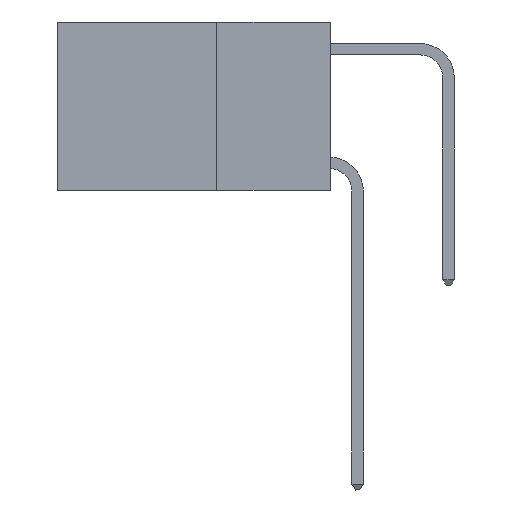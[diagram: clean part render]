
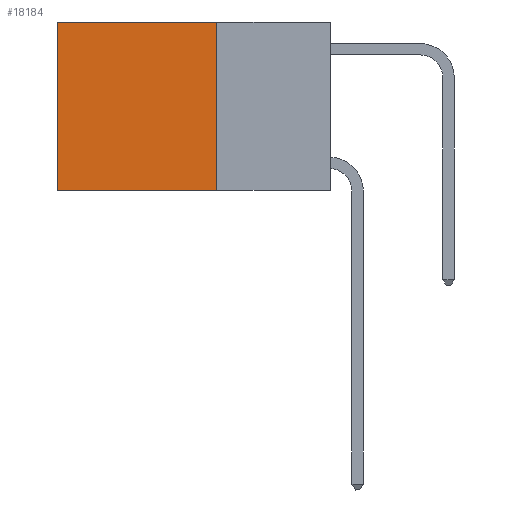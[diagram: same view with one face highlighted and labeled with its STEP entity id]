
A CAD part, left-side view. The second image highlights one B-rep face of the part: STEP entity #18184.
In plain terms, the highlighted planar face has unit normal (-1, 0, 0).
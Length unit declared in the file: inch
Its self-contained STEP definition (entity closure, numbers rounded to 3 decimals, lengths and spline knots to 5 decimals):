
#187 = ORIENTED_EDGE ( 'NONE', *, *, #11373, .F. ) ;
#1562 = VECTOR ( 'NONE', #7530, 39.37008 ) ;
#2436 = VERTEX_POINT ( 'NONE', #14082 ) ;
#2624 = AXIS2_PLACEMENT_3D ( 'NONE', #4639, #6409, #18191 ) ;
#2731 = EDGE_CURVE ( 'NONE', #2436, #19202, #10672, .T. ) ;
#3174 = EDGE_CURVE ( 'NONE', #18540, #13599, #18508, .T. ) ;
#4070 = CARTESIAN_POINT ( 'NONE',  ( 0.2625, 0.6, 0. ) ) ;
#4639 = CARTESIAN_POINT ( 'NONE',  ( 0.2625, 0.25, 0. ) ) ;
#4777 = DIRECTION ( 'NONE',  ( 0., 1., 0. ) ) ;
#5534 = DIRECTION ( 'NONE',  ( 0., 1., 0. ) ) ;
#6160 = VECTOR ( 'NONE', #4777, 39.37008 ) ;
#6291 = LINE ( 'NONE', #4070, #1562 ) ;
#6409 = DIRECTION ( 'NONE',  ( 1., 0., 0. ) ) ;
#7530 = DIRECTION ( 'NONE',  ( 0., 0., -1. ) ) ;
#9052 = VECTOR ( 'NONE', #5534, 39.37008 ) ;
#9371 = CARTESIAN_POINT ( 'NONE',  ( 0.2625, 0.6, -0.37 ) ) ;
#10672 = LINE ( 'NONE', #13339, #6160 ) ;
#10936 = EDGE_LOOP ( 'NONE', ( #17545, #14398, #187, #19787 ) ) ;
#11373 = EDGE_CURVE ( 'NONE', #2436, #18540, #20338, .T. ) ;
#13339 = CARTESIAN_POINT ( 'NONE',  ( 0.2625, 0.25, 0. ) ) ;
#13599 = VERTEX_POINT ( 'NONE', #9371 ) ;
#13996 = CARTESIAN_POINT ( 'NONE',  ( 0.2625, 0.25, -0.37 ) ) ;
#14082 = CARTESIAN_POINT ( 'NONE',  ( 0.2625, 0.25, 0. ) ) ;
#14398 = ORIENTED_EDGE ( 'NONE', *, *, #3174, .F. ) ;
#14642 = FACE_OUTER_BOUND ( 'NONE', #10936, .T. ) ;
#14788 = PLANE ( 'NONE',  #2624 ) ;
#15627 = CARTESIAN_POINT ( 'NONE',  ( 0.2625, 0.25, 0. ) ) ;
#16751 = CARTESIAN_POINT ( 'NONE',  ( 0.2625, 0.6, 0. ) ) ;
#17252 = CARTESIAN_POINT ( 'NONE',  ( 0.2625, 0.25, -0.37 ) ) ;
#17310 = DIRECTION ( 'NONE',  ( 0., 0., -1. ) ) ;
#17545 = ORIENTED_EDGE ( 'NONE', *, *, #19544, .T. ) ;
#18184 = ADVANCED_FACE ( 'NONE', ( #14642 ), #14788, .F. ) ;
#18191 = DIRECTION ( 'NONE',  ( 0., 0., -1. ) ) ;
#18508 = LINE ( 'NONE', #17252, #9052 ) ;
#18540 = VERTEX_POINT ( 'NONE', #13996 ) ;
#19202 = VERTEX_POINT ( 'NONE', #16751 ) ;
#19544 = EDGE_CURVE ( 'NONE', #19202, #13599, #6291, .T. ) ;
#19787 = ORIENTED_EDGE ( 'NONE', *, *, #2731, .T. ) ;
#19808 = VECTOR ( 'NONE', #17310, 39.37008 ) ;
#20338 = LINE ( 'NONE', #15627, #19808 ) ;
